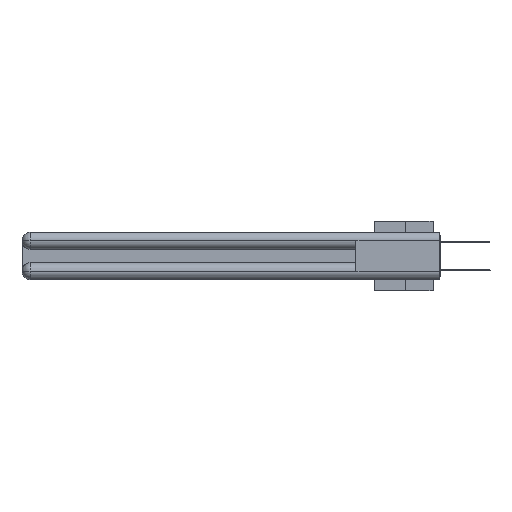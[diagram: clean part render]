
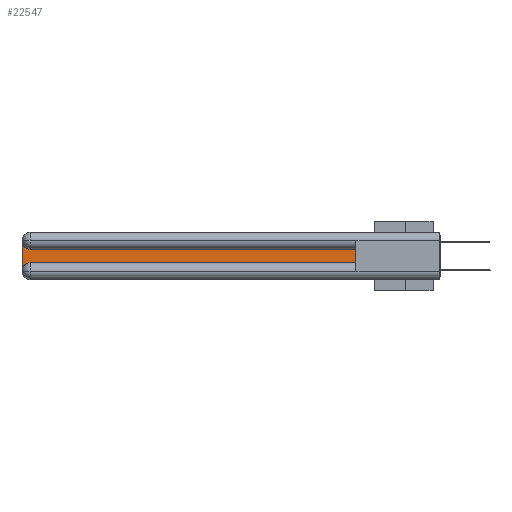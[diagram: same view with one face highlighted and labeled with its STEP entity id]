
A CAD part, left-side view. The second image highlights one B-rep face of the part: STEP entity #22547.
In plain terms, the highlighted planar face has unit normal (-1, 0, 0).
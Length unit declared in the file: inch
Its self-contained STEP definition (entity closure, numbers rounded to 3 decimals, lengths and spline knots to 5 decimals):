
#865 = AXIS2_PLACEMENT_3D ( 'NONE', #30263, #18247, #13695 ) ;
#1671 = CARTESIAN_POINT ( 'NONE',  ( 0.075, 0.6, -0.2175 ) ) ;
#1824 = DIRECTION ( 'NONE',  ( 0., 0., 1. ) ) ;
#2065 = CARTESIAN_POINT ( 'NONE',  ( 0.075, 3., -0.2175 ) ) ;
#2160 = EDGE_CURVE ( 'NONE', #6737, #28122, #29977, .T. ) ;
#2978 = VECTOR ( 'NONE', #1824, 39.37008 ) ;
#3690 = VECTOR ( 'NONE', #30737, 39.37008 ) ;
#4163 = ORIENTED_EDGE ( 'NONE', *, *, #26275, .T. ) ;
#6144 = ORIENTED_EDGE ( 'NONE', *, *, #17944, .T. ) ;
#6181 = VECTOR ( 'NONE', #26418, 39.37008 ) ;
#6737 = VERTEX_POINT ( 'NONE', #12565 ) ;
#6761 = VERTEX_POINT ( 'NONE', #8632 ) ;
#7394 = LINE ( 'NONE', #16886, #6181 ) ;
#7539 = DIRECTION ( 'NONE',  ( 1., 0., 0. ) ) ;
#8632 = CARTESIAN_POINT ( 'NONE',  ( 0.075, 3., -0.0625 ) ) ;
#8650 = LINE ( 'NONE', #1671, #2978 ) ;
#8912 = DIRECTION ( 'NONE',  ( 0., 0., -1. ) ) ;
#9203 = EDGE_CURVE ( 'NONE', #16647, #26306, #17776, .T. ) ;
#9502 = CARTESIAN_POINT ( 'NONE',  ( 0.075, 3., -0.2775 ) ) ;
#9506 = LINE ( 'NONE', #2065, #3690 ) ;
#9792 = CARTESIAN_POINT ( 'NONE',  ( 0.075, 0.6, -0.2175 ) ) ;
#11275 = AXIS2_PLACEMENT_3D ( 'NONE', #28909, #7539, #17034 ) ;
#11446 = CIRCLE ( 'NONE', #16438, 0.06 ) ;
#12565 = CARTESIAN_POINT ( 'NONE',  ( 0.075, 0.6, -0.1225 ) ) ;
#13498 = EDGE_CURVE ( 'NONE', #15394, #6737, #8650, .T. ) ;
#13695 = DIRECTION ( 'NONE',  ( 0., 0., -1. ) ) ;
#15394 = VERTEX_POINT ( 'NONE', #9792 ) ;
#16074 = CARTESIAN_POINT ( 'NONE',  ( 0.075, 2.94, -0.2175 ) ) ;
#16218 = ORIENTED_EDGE ( 'NONE', *, *, #2160, .T. ) ;
#16261 = VECTOR ( 'NONE', #24984, 39.37008 ) ;
#16438 = AXIS2_PLACEMENT_3D ( 'NONE', #30449, #26072, #8912 ) ;
#16647 = VERTEX_POINT ( 'NONE', #9502 ) ;
#16886 = CARTESIAN_POINT ( 'NONE',  ( 0.075, 0.6, -0.2175 ) ) ;
#17034 = DIRECTION ( 'NONE',  ( 0., 0., -1. ) ) ;
#17742 = ORIENTED_EDGE ( 'NONE', *, *, #13498, .T. ) ;
#17776 = CIRCLE ( 'NONE', #865, 0.06 ) ;
#17944 = EDGE_CURVE ( 'NONE', #6761, #16647, #9506, .T. ) ;
#18247 = DIRECTION ( 'NONE',  ( 1., 0., 0. ) ) ;
#18821 = CARTESIAN_POINT ( 'NONE',  ( 0.075, 2.94, -0.1225 ) ) ;
#21005 = EDGE_LOOP ( 'NONE', ( #16218, #4163, #6144, #22436, #23034, #17742 ) ) ;
#22436 = ORIENTED_EDGE ( 'NONE', *, *, #9203, .T. ) ;
#22547 = ADVANCED_FACE ( 'NONE', ( #26114 ), #25969, .F. ) ;
#23034 = ORIENTED_EDGE ( 'NONE', *, *, #30001, .T. ) ;
#24984 = DIRECTION ( 'NONE',  ( 0., 1., 0. ) ) ;
#25969 = PLANE ( 'NONE',  #11275 ) ;
#26072 = DIRECTION ( 'NONE',  ( 1., 0., 0. ) ) ;
#26114 = FACE_OUTER_BOUND ( 'NONE', #21005, .T. ) ;
#26275 = EDGE_CURVE ( 'NONE', #28122, #6761, #11446, .T. ) ;
#26306 = VERTEX_POINT ( 'NONE', #16074 ) ;
#26418 = DIRECTION ( 'NONE',  ( 0., -1., 0. ) ) ;
#27503 = CARTESIAN_POINT ( 'NONE',  ( 0.075, 0.6, -0.1225 ) ) ;
#28122 = VERTEX_POINT ( 'NONE', #18821 ) ;
#28909 = CARTESIAN_POINT ( 'NONE',  ( 0.075, 3., -0.1225 ) ) ;
#29977 = LINE ( 'NONE', #27503, #16261 ) ;
#30001 = EDGE_CURVE ( 'NONE', #26306, #15394, #7394, .T. ) ;
#30263 = CARTESIAN_POINT ( 'NONE',  ( 0.075, 2.94, -0.2775 ) ) ;
#30449 = CARTESIAN_POINT ( 'NONE',  ( 0.075, 2.94, -0.0625 ) ) ;
#30737 = DIRECTION ( 'NONE',  ( 0., 0., -1. ) ) ;
